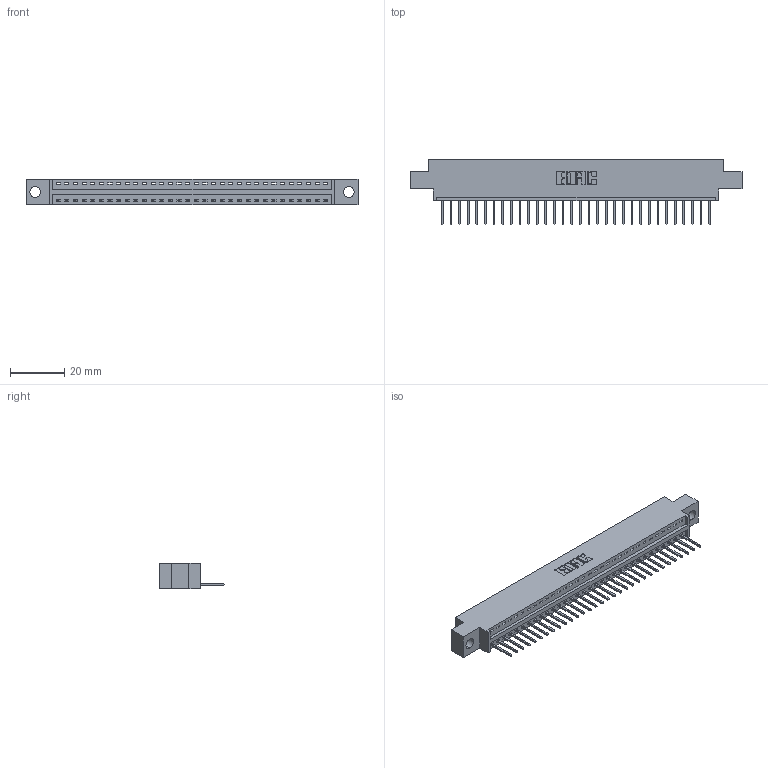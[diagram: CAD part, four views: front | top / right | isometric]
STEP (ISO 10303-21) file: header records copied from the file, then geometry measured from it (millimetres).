
FILE_DESCRIPTION (( 'STEP AP203' ), '1' );
FILE_NAME ('346-032-526-604.STEP', '2018-08-22T08:54:45', ( '' ), ( '' ), 'SwSTEP 2.0', 'SolidWorks 2016', '' );
FILE_SCHEMA (( 'CONFIG_CONTROL_DESIGN' ));
Length unit declared in the file: inch
Products named in the file (3): 346 Part_0.170 Offset - 0.156 Dia-TH; 345-292-001_345-293-126; 346-032-526-604
Assembly tree (33 placements, depth 2):
  346-032-526-604
    346 Part_0.170 Offset - 0.156 Dia-TH
    345-292-001_345-293-126  x32
Bounding box: 122.17 x 24.13 x 9.4 mm (x, y, z)
Volume: 11357.9 mm3; surface area: 14022.1 mm2
Topology: 33 solids, 33 shells, 1982 faces, 5973 edges, 3938 vertices
Faces by surface type: plane 1360, cylinder 622
Entity records: 21359 total; most frequent: CARTESIAN_POINT 3672, ORIENTED_EDGE 3638, DIRECTION 3251, EDGE_CURVE 1819, LINE 1559, VECTOR 1559, VERTEX_POINT 1210, AXIS2_PLACEMENT_3D 846
